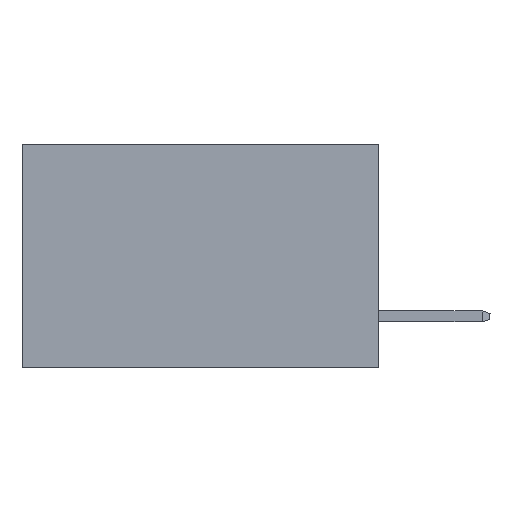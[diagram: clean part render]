
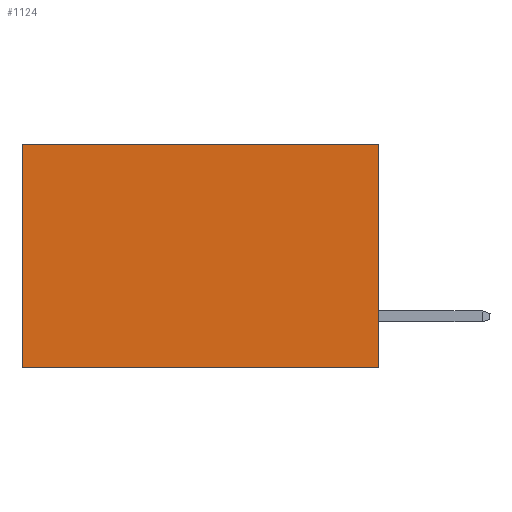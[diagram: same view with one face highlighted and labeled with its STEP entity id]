
A CAD part, left-side view. The second image highlights one B-rep face of the part: STEP entity #1124.
In plain terms, the highlighted planar face has unit normal (-1, 0, 0).
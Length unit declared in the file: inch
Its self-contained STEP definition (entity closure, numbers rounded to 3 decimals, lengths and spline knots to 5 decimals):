
#159 = CARTESIAN_POINT ( 'NONE',  ( 0.277, 0., -0.37 ) ) ;
#1124 = ADVANCED_FACE ( 'NONE', ( #9662 ), #1544, .F. ) ;
#1544 = PLANE ( 'NONE',  #7323 ) ;
#1921 = EDGE_CURVE ( 'NONE', #4158, #2469, #2025, .T. ) ;
#2025 = LINE ( 'NONE', #7465, #2268 ) ;
#2200 = ORIENTED_EDGE ( 'NONE', *, *, #7877, .T. ) ;
#2202 = VERTEX_POINT ( 'NONE', #5093 ) ;
#2268 = VECTOR ( 'NONE', #3717, 39.37008 ) ;
#2469 = VERTEX_POINT ( 'NONE', #6177 ) ;
#2489 = DIRECTION ( 'NONE',  ( 0., 0., -1. ) ) ;
#3500 = LINE ( 'NONE', #8958, #7244 ) ;
#3594 = EDGE_CURVE ( 'NONE', #2202, #4158, #8731, .T. ) ;
#3717 = DIRECTION ( 'NONE',  ( 0., 1., 0. ) ) ;
#4158 = VERTEX_POINT ( 'NONE', #7319 ) ;
#4360 = LINE ( 'NONE', #9829, #8546 ) ;
#5057 = DIRECTION ( 'NONE',  ( 0., 0., -1. ) ) ;
#5093 = CARTESIAN_POINT ( 'NONE',  ( 0.277, 0., 0. ) ) ;
#6124 = ORIENTED_EDGE ( 'NONE', *, *, #7712, .T. ) ;
#6177 = CARTESIAN_POINT ( 'NONE',  ( 0.277, 0.59, -0.37 ) ) ;
#6347 = CARTESIAN_POINT ( 'NONE',  ( 0.277, 0., -0.37 ) ) ;
#6392 = DIRECTION ( 'NONE',  ( 1., 0., 0. ) ) ;
#6668 = DIRECTION ( 'NONE',  ( 0., 0., -1. ) ) ;
#6944 = VECTOR ( 'NONE', #2489, 39.37008 ) ;
#6977 = EDGE_LOOP ( 'NONE', ( #6124, #8230, #10172, #2200 ) ) ;
#7244 = VECTOR ( 'NONE', #5057, 39.37008 ) ;
#7319 = CARTESIAN_POINT ( 'NONE',  ( 0.277, 0., -0.37 ) ) ;
#7323 = AXIS2_PLACEMENT_3D ( 'NONE', #6347, #6392, #6668 ) ;
#7465 = CARTESIAN_POINT ( 'NONE',  ( 0.277, 0., -0.37 ) ) ;
#7712 = EDGE_CURVE ( 'NONE', #7737, #2469, #3500, .T. ) ;
#7737 = VERTEX_POINT ( 'NONE', #8236 ) ;
#7877 = EDGE_CURVE ( 'NONE', #2202, #7737, #4360, .T. ) ;
#8230 = ORIENTED_EDGE ( 'NONE', *, *, #1921, .F. ) ;
#8236 = CARTESIAN_POINT ( 'NONE',  ( 0.277, 0.59, 0. ) ) ;
#8348 = DIRECTION ( 'NONE',  ( 0., 1., 0. ) ) ;
#8546 = VECTOR ( 'NONE', #8348, 39.37008 ) ;
#8731 = LINE ( 'NONE', #159, #6944 ) ;
#8958 = CARTESIAN_POINT ( 'NONE',  ( 0.277, 0.59, -0.37 ) ) ;
#9662 = FACE_OUTER_BOUND ( 'NONE', #6977, .T. ) ;
#9829 = CARTESIAN_POINT ( 'NONE',  ( 0.277, 0., 0. ) ) ;
#10172 = ORIENTED_EDGE ( 'NONE', *, *, #3594, .F. ) ;
